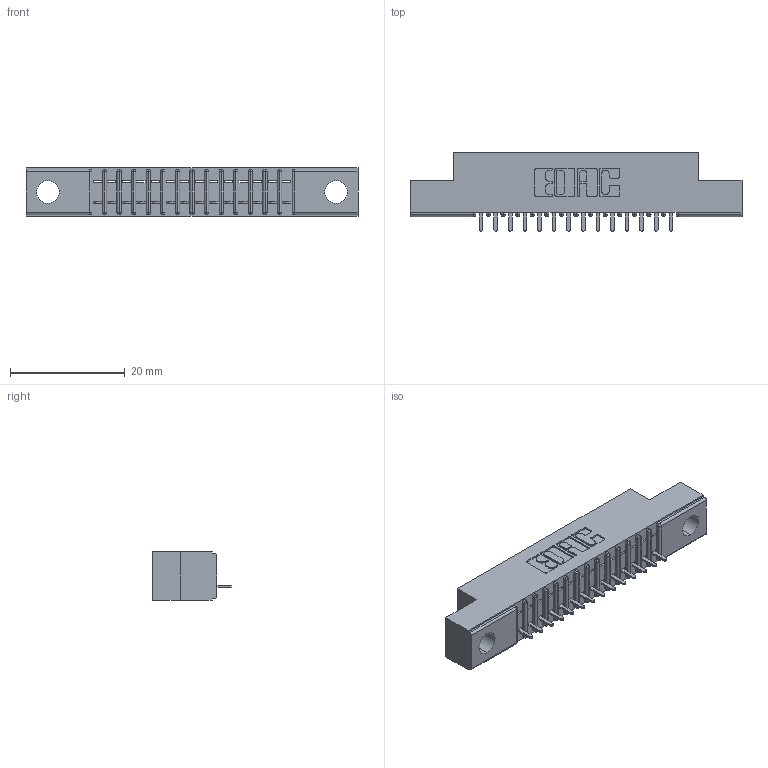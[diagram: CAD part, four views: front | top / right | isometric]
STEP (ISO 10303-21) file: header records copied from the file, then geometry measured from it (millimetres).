
FILE_DESCRIPTION (( 'STEP AP203' ), '1' );
FILE_NAME ('391-014-524-104.STEP', '2018-08-08T17:09:38', ( '' ), ( '' ), 'SwSTEP 2.0', 'SolidWorks 2016', '' );
FILE_SCHEMA (( 'CONFIG_CONTROL_DESIGN' ));
Length unit declared in the file: inch
Products named in the file (3): 391-014-524-104; 341 Part_.156 (3.96) Dia Mounting Holes; 341-292-001_341-292-124
Assembly tree (15 placements, depth 2):
  391-014-524-104
    341 Part_.156 (3.96) Dia Mounting Holes
    341-292-001_341-292-124  x14
Bounding box: 57.78 x 13.64 x 8.38 mm (x, y, z)
Volume: 3104.1 mm3; surface area: 5198.7 mm2
Topology: 15 solids, 15 shells, 1278 faces, 3670 edges, 2358 vertices
Faces by surface type: plane 796, cylinder 426, sphere 30, torus 26
Entity records: 20643 total; most frequent: CARTESIAN_POINT 3498, ORIENTED_EDGE 3484, DIRECTION 3392, EDGE_CURVE 1742, VECTOR 1384, LINE 1384, VERTEX_POINT 1110, AXIS2_PLACEMENT_3D 1004
